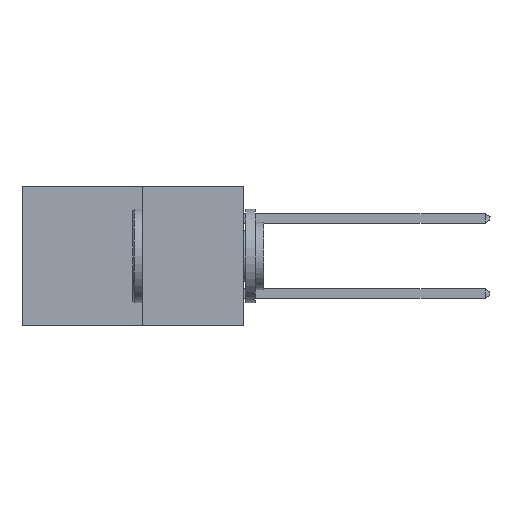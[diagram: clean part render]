
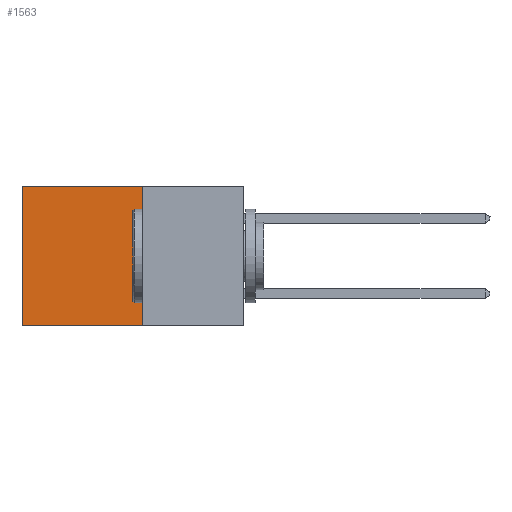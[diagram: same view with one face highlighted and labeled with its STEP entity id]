
A CAD part, left-side view. The second image highlights one B-rep face of the part: STEP entity #1563.
In plain terms, the highlighted planar face has unit normal (-1, 0, 0).
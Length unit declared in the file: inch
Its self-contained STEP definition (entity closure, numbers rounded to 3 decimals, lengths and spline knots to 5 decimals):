
#11 = DIRECTION ( 'NONE',  ( 1., 0., 0. ) ) ;
#45 = CARTESIAN_POINT ( 'NONE',  ( 0.277, 0.27, -0.37 ) ) ;
#292 = EDGE_CURVE ( 'NONE', #1385, #9549, #2585, .T. ) ;
#855 = DIRECTION ( 'NONE',  ( 0., 1., 0. ) ) ;
#1105 = CARTESIAN_POINT ( 'NONE',  ( 0.277, 0.27, 0. ) ) ;
#1385 = VERTEX_POINT ( 'NONE', #2072 ) ;
#1563 = ADVANCED_FACE ( 'NONE', ( #3068 ), #4483, .F. ) ;
#1605 = DIRECTION ( 'NONE',  ( 0., 0., -1. ) ) ;
#2072 = CARTESIAN_POINT ( 'NONE',  ( 0.277, 0.59, 0. ) ) ;
#2177 = VECTOR ( 'NONE', #855, 39.37008 ) ;
#2521 = LINE ( 'NONE', #1105, #2177 ) ;
#2585 = LINE ( 'NONE', #9085, #11110 ) ;
#2989 = ORIENTED_EDGE ( 'NONE', *, *, #3933, .F. ) ;
#3068 = FACE_OUTER_BOUND ( 'NONE', #5725, .T. ) ;
#3285 = EDGE_CURVE ( 'NONE', #7364, #1385, #2521, .T. ) ;
#3823 = ORIENTED_EDGE ( 'NONE', *, *, #5160, .F. ) ;
#3933 = EDGE_CURVE ( 'NONE', #7364, #9722, #5470, .T. ) ;
#3994 = CARTESIAN_POINT ( 'NONE',  ( 0.277, 0.27, -0.37 ) ) ;
#4355 = DIRECTION ( 'NONE',  ( 0., 1., 0. ) ) ;
#4483 = PLANE ( 'NONE',  #5801 ) ;
#4622 = VECTOR ( 'NONE', #4355, 39.37008 ) ;
#4660 = DIRECTION ( 'NONE',  ( 0., 0., -1. ) ) ;
#5160 = EDGE_CURVE ( 'NONE', #9722, #9549, #12438, .T. ) ;
#5470 = LINE ( 'NONE', #9481, #6148 ) ;
#5552 = CARTESIAN_POINT ( 'NONE',  ( 0.277, 0.27, 0. ) ) ;
#5677 = DIRECTION ( 'NONE',  ( 0., 0., -1. ) ) ;
#5725 = EDGE_LOOP ( 'NONE', ( #13397, #3823, #2989, #11668 ) ) ;
#5801 = AXIS2_PLACEMENT_3D ( 'NONE', #45, #11, #4660 ) ;
#6148 = VECTOR ( 'NONE', #1605, 39.37008 ) ;
#7364 = VERTEX_POINT ( 'NONE', #5552 ) ;
#8179 = CARTESIAN_POINT ( 'NONE',  ( 0.277, 0.27, -0.37 ) ) ;
#9085 = CARTESIAN_POINT ( 'NONE',  ( 0.277, 0.59, -0.37 ) ) ;
#9481 = CARTESIAN_POINT ( 'NONE',  ( 0.277, 0.27, -0.37 ) ) ;
#9549 = VERTEX_POINT ( 'NONE', #13264 ) ;
#9722 = VERTEX_POINT ( 'NONE', #8179 ) ;
#11110 = VECTOR ( 'NONE', #5677, 39.37008 ) ;
#11668 = ORIENTED_EDGE ( 'NONE', *, *, #3285, .T. ) ;
#12438 = LINE ( 'NONE', #3994, #4622 ) ;
#13264 = CARTESIAN_POINT ( 'NONE',  ( 0.277, 0.59, -0.37 ) ) ;
#13397 = ORIENTED_EDGE ( 'NONE', *, *, #292, .T. ) ;
